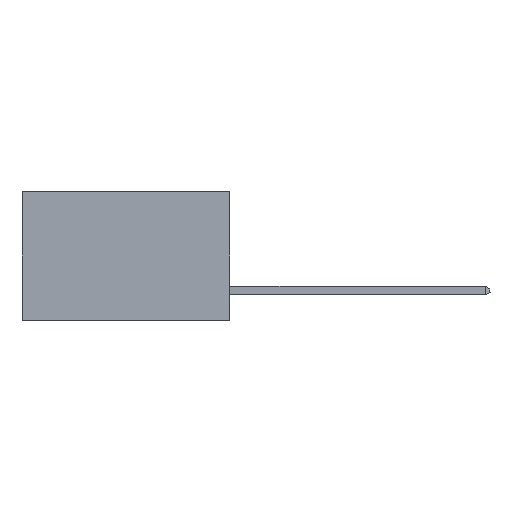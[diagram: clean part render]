
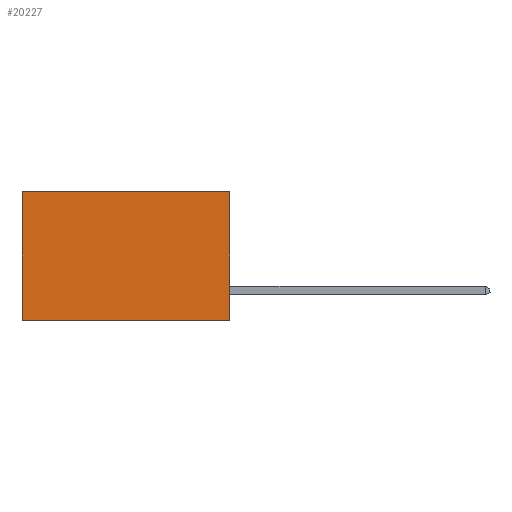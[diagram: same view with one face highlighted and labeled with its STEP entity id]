
A CAD part, left-side view. The second image highlights one B-rep face of the part: STEP entity #20227.
In plain terms, the highlighted planar face has unit normal (-1, 0, 0).
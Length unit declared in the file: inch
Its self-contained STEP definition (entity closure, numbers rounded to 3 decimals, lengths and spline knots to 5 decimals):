
#460 = AXIS2_PLACEMENT_3D ( 'NONE', #22772, #6466, #22542 ) ;
#1070 = CARTESIAN_POINT ( 'NONE',  ( 0.298, 0.6, 0. ) ) ;
#1244 = CARTESIAN_POINT ( 'NONE',  ( 0.298, 0., 0. ) ) ;
#1756 = CARTESIAN_POINT ( 'NONE',  ( 0.298, 0., -0.37 ) ) ;
#1772 = CARTESIAN_POINT ( 'NONE',  ( 0.298, 0., 0. ) ) ;
#2240 = CARTESIAN_POINT ( 'NONE',  ( 0.298, 0., -0.37 ) ) ;
#2802 = DIRECTION ( 'NONE',  ( 0., 1., 0. ) ) ;
#2865 = DIRECTION ( 'NONE',  ( 0., 0., -1. ) ) ;
#5402 = DIRECTION ( 'NONE',  ( 0., 0., -1. ) ) ;
#5832 = ORIENTED_EDGE ( 'NONE', *, *, #16053, .T. ) ;
#6054 = EDGE_CURVE ( 'NONE', #14381, #13769, #15044, .T. ) ;
#6466 = DIRECTION ( 'NONE',  ( 1., 0., 0. ) ) ;
#7577 = ORIENTED_EDGE ( 'NONE', *, *, #7940, .F. ) ;
#7780 = CARTESIAN_POINT ( 'NONE',  ( 0.298, 0.6, -0.37 ) ) ;
#7940 = EDGE_CURVE ( 'NONE', #14381, #16158, #20875, .T. ) ;
#10428 = VECTOR ( 'NONE', #14875, 39.37008 ) ;
#10855 = EDGE_LOOP ( 'NONE', ( #5832, #19285, #7577, #21447 ) ) ;
#12336 = VERTEX_POINT ( 'NONE', #7780 ) ;
#12687 = VECTOR ( 'NONE', #5402, 39.37008 ) ;
#12763 = CARTESIAN_POINT ( 'NONE',  ( 0.298, 0.6, 0. ) ) ;
#13050 = VECTOR ( 'NONE', #2865, 39.37008 ) ;
#13722 = PLANE ( 'NONE',  #460 ) ;
#13769 = VERTEX_POINT ( 'NONE', #12763 ) ;
#14381 = VERTEX_POINT ( 'NONE', #19914 ) ;
#14875 = DIRECTION ( 'NONE',  ( 0., 1., 0. ) ) ;
#15044 = LINE ( 'NONE', #1244, #17565 ) ;
#16053 = EDGE_CURVE ( 'NONE', #13769, #12336, #21498, .T. ) ;
#16158 = VERTEX_POINT ( 'NONE', #1756 ) ;
#17565 = VECTOR ( 'NONE', #2802, 39.37008 ) ;
#18906 = EDGE_CURVE ( 'NONE', #16158, #12336, #19402, .T. ) ;
#19285 = ORIENTED_EDGE ( 'NONE', *, *, #18906, .F. ) ;
#19402 = LINE ( 'NONE', #2240, #10428 ) ;
#19914 = CARTESIAN_POINT ( 'NONE',  ( 0.298, 0., 0. ) ) ;
#20227 = ADVANCED_FACE ( 'NONE', ( #22416 ), #13722, .F. ) ;
#20875 = LINE ( 'NONE', #1772, #12687 ) ;
#21447 = ORIENTED_EDGE ( 'NONE', *, *, #6054, .T. ) ;
#21498 = LINE ( 'NONE', #1070, #13050 ) ;
#22416 = FACE_OUTER_BOUND ( 'NONE', #10855, .T. ) ;
#22542 = DIRECTION ( 'NONE',  ( 0., 0., -1. ) ) ;
#22772 = CARTESIAN_POINT ( 'NONE',  ( 0.298, 0., 0. ) ) ;
